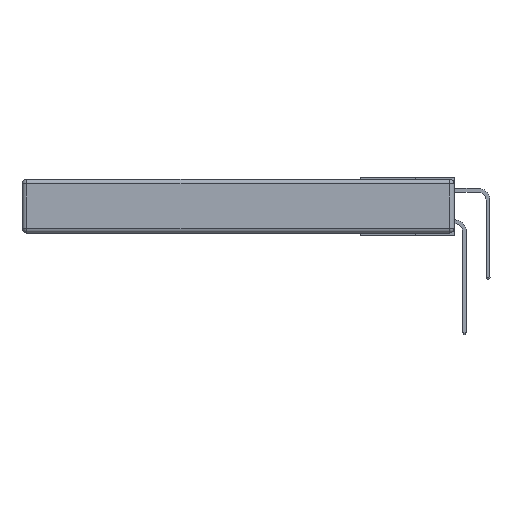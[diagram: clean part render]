
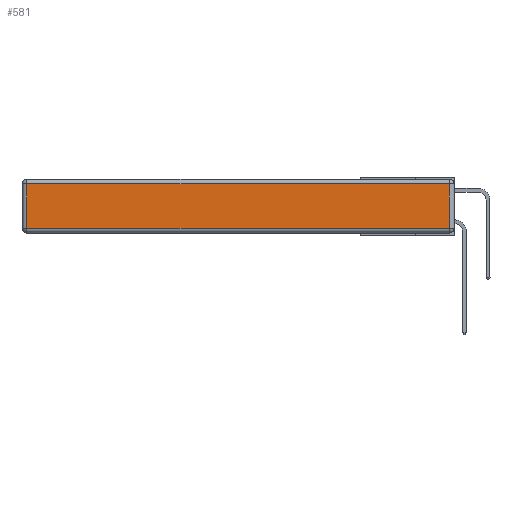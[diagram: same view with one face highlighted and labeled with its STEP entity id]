
A CAD part, left-side view. The second image highlights one B-rep face of the part: STEP entity #581.
In plain terms, the highlighted planar face has unit normal (-1, 0, 0).
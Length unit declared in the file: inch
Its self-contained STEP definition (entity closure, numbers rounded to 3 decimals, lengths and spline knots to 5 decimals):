
#581 = ADVANCED_FACE ( 'NONE', ( #9048 ), #14439, .T. ) ;
#645 = LINE ( 'NONE', #17582, #26197 ) ;
#735 = DIRECTION ( 'NONE',  ( 0., 0., 1. ) ) ;
#1247 = LINE ( 'NONE', #9398, #27434 ) ;
#1598 = CARTESIAN_POINT ( 'NONE',  ( 0., 0., -0.343 ) ) ;
#1636 = EDGE_CURVE ( 'NONE', #5845, #18526, #10313, .T. ) ;
#2877 = VERTEX_POINT ( 'NONE', #13680 ) ;
#3184 = CARTESIAN_POINT ( 'NONE',  ( 0., 0.03, -0.03 ) ) ;
#4502 = EDGE_CURVE ( 'NONE', #8433, #2877, #1247, .T. ) ;
#5845 = VERTEX_POINT ( 'NONE', #3184 ) ;
#8433 = VERTEX_POINT ( 'NONE', #23269 ) ;
#9048 = FACE_OUTER_BOUND ( 'NONE', #10832, .T. ) ;
#9398 = CARTESIAN_POINT ( 'NONE',  ( 0., 0., -0.313 ) ) ;
#10313 = LINE ( 'NONE', #26208, #19018 ) ;
#10754 = EDGE_CURVE ( 'NONE', #2877, #5845, #645, .T. ) ;
#10758 = ORIENTED_EDGE ( 'NONE', *, *, #1636, .T. ) ;
#10832 = EDGE_LOOP ( 'NONE', ( #11779, #25152, #10758, #18414 ) ) ;
#11058 = AXIS2_PLACEMENT_3D ( 'NONE', #1598, #18809, #16510 ) ;
#11272 = DIRECTION ( 'NONE',  ( 0., 1., 0. ) ) ;
#11291 = DIRECTION ( 'NONE',  ( 0., -1., 0. ) ) ;
#11779 = ORIENTED_EDGE ( 'NONE', *, *, #4502, .T. ) ;
#13680 = CARTESIAN_POINT ( 'NONE',  ( 0., 0.03, -0.313 ) ) ;
#14439 = PLANE ( 'NONE',  #11058 ) ;
#15423 = DIRECTION ( 'NONE',  ( 0., 0., -1. ) ) ;
#16428 = EDGE_CURVE ( 'NONE', #18526, #8433, #22311, .T. ) ;
#16510 = DIRECTION ( 'NONE',  ( 0., 0., 1. ) ) ;
#17582 = CARTESIAN_POINT ( 'NONE',  ( 0., 0.03, -0.343 ) ) ;
#17905 = CARTESIAN_POINT ( 'NONE',  ( 0., 2.72, -0.03 ) ) ;
#18414 = ORIENTED_EDGE ( 'NONE', *, *, #16428, .T. ) ;
#18526 = VERTEX_POINT ( 'NONE', #17905 ) ;
#18809 = DIRECTION ( 'NONE',  ( -1., 0., 0. ) ) ;
#19018 = VECTOR ( 'NONE', #11272, 39.37008 ) ;
#19860 = CARTESIAN_POINT ( 'NONE',  ( 0., 2.72, -0.343 ) ) ;
#22311 = LINE ( 'NONE', #19860, #24308 ) ;
#23269 = CARTESIAN_POINT ( 'NONE',  ( 0., 2.72, -0.313 ) ) ;
#24308 = VECTOR ( 'NONE', #15423, 39.37008 ) ;
#25152 = ORIENTED_EDGE ( 'NONE', *, *, #10754, .T. ) ;
#26197 = VECTOR ( 'NONE', #735, 39.37008 ) ;
#26208 = CARTESIAN_POINT ( 'NONE',  ( 0., 2.75, -0.03 ) ) ;
#27434 = VECTOR ( 'NONE', #11291, 39.37008 ) ;
